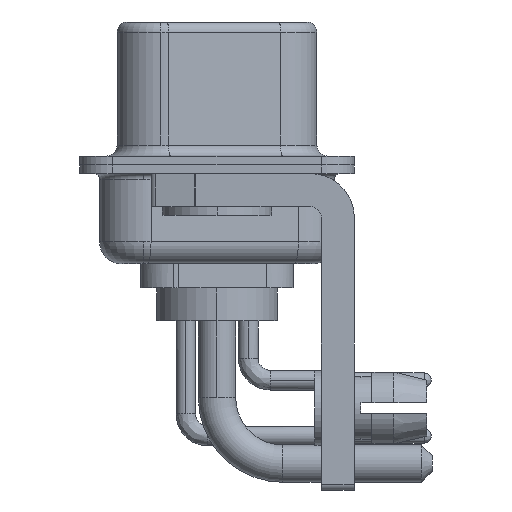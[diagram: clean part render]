
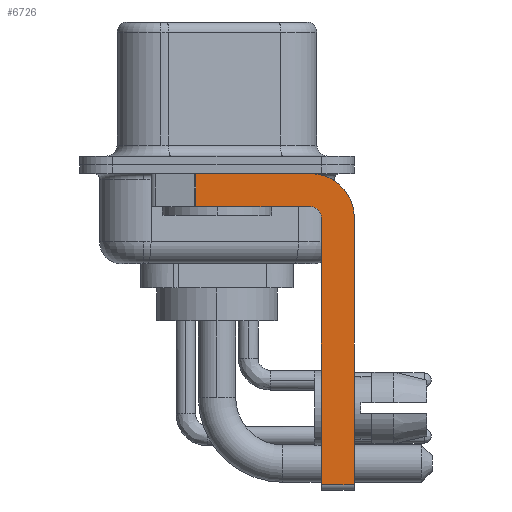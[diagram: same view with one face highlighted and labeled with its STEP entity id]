
A CAD part, left-side view. The second image highlights one B-rep face of the part: STEP entity #6726.
In plain terms, the highlighted planar face has unit normal (-1, 0, 0).
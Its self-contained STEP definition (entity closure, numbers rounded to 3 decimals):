
#48 = DIRECTION ( 'NONE',  ( 0., -1., 0. ) ) ;
#87 = PLANE ( 'NONE',  #20962 ) ;
#122 = CARTESIAN_POINT ( 'NONE',  ( -2.9, -4.75, -2.4 ) ) ;
#346 = EDGE_CURVE ( 'NONE', #7438, #11156, #21705, .T. ) ;
#1216 = VERTEX_POINT ( 'NONE', #8095 ) ;
#1257 = CARTESIAN_POINT ( 'NONE',  ( -2.9, 0.978, -0.4 ) ) ;
#1476 = CARTESIAN_POINT ( 'NONE',  ( -2.9, -4.25, -2.4 ) ) ;
#1840 = DIRECTION ( 'NONE',  ( 1., 0., 0. ) ) ;
#2234 = FACE_OUTER_BOUND ( 'NONE', #18612, .T. ) ;
#3149 = VERTEX_POINT ( 'NONE', #19498 ) ;
#3639 = CARTESIAN_POINT ( 'NONE',  ( -2.9, 0.978, -1.9 ) ) ;
#5257 = ORIENTED_EDGE ( 'NONE', *, *, #14508, .F. ) ;
#5869 = EDGE_CURVE ( 'NONE', #7438, #3149, #22222, .T. ) ;
#6054 = EDGE_CURVE ( 'NONE', #3149, #11250, #22698, .T. ) ;
#6210 = VERTEX_POINT ( 'NONE', #122 ) ;
#6679 = ORIENTED_EDGE ( 'NONE', *, *, #24020, .F. ) ;
#6726 = ADVANCED_FACE ( 'NONE', ( #2234 ), #87, .F. ) ;
#7407 = VECTOR ( 'NONE', #7600, 1000. ) ;
#7438 = VERTEX_POINT ( 'NONE', #1257 ) ;
#7576 = LINE ( 'NONE', #26226, #7935 ) ;
#7600 = DIRECTION ( 'NONE',  ( 0., 1., 0. ) ) ;
#7700 = CIRCLE ( 'NONE', #17254, 0.5 ) ;
#7927 = CARTESIAN_POINT ( 'NONE',  ( -2.9, 3., -0.4 ) ) ;
#7935 = VECTOR ( 'NONE', #20372, 1000. ) ;
#8095 = CARTESIAN_POINT ( 'NONE',  ( -2.9, -6.25, -14.55 ) ) ;
#8787 = CARTESIAN_POINT ( 'NONE',  ( -2.9, -6.25, -2.4 ) ) ;
#9213 = AXIS2_PLACEMENT_3D ( 'NONE', #1476, #23934, #15890 ) ;
#10124 = CARTESIAN_POINT ( 'NONE',  ( -2.9, -4.75, -14.55 ) ) ;
#10444 = CARTESIAN_POINT ( 'NONE',  ( -2.9, -6.25, -2.4 ) ) ;
#11156 = VERTEX_POINT ( 'NONE', #3639 ) ;
#11174 = CARTESIAN_POINT ( 'NONE',  ( -2.9, -4.25, -1.9 ) ) ;
#11250 = VERTEX_POINT ( 'NONE', #10444 ) ;
#11798 = ORIENTED_EDGE ( 'NONE', *, *, #16405, .F. ) ;
#12234 = VECTOR ( 'NONE', #48, 1000. ) ;
#13249 = CARTESIAN_POINT ( 'NONE',  ( -2.9, 0.978, -1.9 ) ) ;
#14508 = EDGE_CURVE ( 'NONE', #6210, #23359, #7700, .T. ) ;
#14541 = LINE ( 'NONE', #18670, #16910 ) ;
#14832 = ORIENTED_EDGE ( 'NONE', *, *, #6054, .F. ) ;
#15890 = DIRECTION ( 'NONE',  ( 0., 0., -1. ) ) ;
#16405 = EDGE_CURVE ( 'NONE', #24233, #6210, #14541, .T. ) ;
#16554 = ORIENTED_EDGE ( 'NONE', *, *, #346, .T. ) ;
#16667 = DIRECTION ( 'NONE',  ( 0., 0., -1. ) ) ;
#16910 = VECTOR ( 'NONE', #23007, 1000. ) ;
#17254 = AXIS2_PLACEMENT_3D ( 'NONE', #18342, #18069, #22569 ) ;
#17603 = ORIENTED_EDGE ( 'NONE', *, *, #25861, .T. ) ;
#18069 = DIRECTION ( 'NONE',  ( -1., 0., 0. ) ) ;
#18144 = VECTOR ( 'NONE', #19416, 1000. ) ;
#18342 = CARTESIAN_POINT ( 'NONE',  ( -2.9, -4.25, -2.4 ) ) ;
#18612 = EDGE_LOOP ( 'NONE', ( #25729, #16554, #6679, #5257, #11798, #17603, #20588, #14832 ) ) ;
#18670 = CARTESIAN_POINT ( 'NONE',  ( -2.9, -4.75, -14.8 ) ) ;
#19051 = EDGE_CURVE ( 'NONE', #11250, #1216, #21045, .T. ) ;
#19416 = DIRECTION ( 'NONE',  ( 0., 0., -1. ) ) ;
#19498 = CARTESIAN_POINT ( 'NONE',  ( -2.9, -4.25, -0.4 ) ) ;
#20372 = DIRECTION ( 'NONE',  ( 0., -1., 0. ) ) ;
#20490 = CARTESIAN_POINT ( 'NONE',  ( -2.9, -4.25, -2.4 ) ) ;
#20588 = ORIENTED_EDGE ( 'NONE', *, *, #19051, .F. ) ;
#20962 = AXIS2_PLACEMENT_3D ( 'NONE', #20490, #1840, #16667 ) ;
#21045 = LINE ( 'NONE', #8787, #18144 ) ;
#21520 = VECTOR ( 'NONE', #25524, 1000. ) ;
#21705 = LINE ( 'NONE', #13249, #21520 ) ;
#22222 = LINE ( 'NONE', #7927, #12234 ) ;
#22569 = DIRECTION ( 'NONE',  ( 0., 0., 1. ) ) ;
#22698 = CIRCLE ( 'NONE', #9213, 2. ) ;
#23007 = DIRECTION ( 'NONE',  ( 0., 0., 1. ) ) ;
#23359 = VERTEX_POINT ( 'NONE', #11174 ) ;
#23934 = DIRECTION ( 'NONE',  ( 1., 0., 0. ) ) ;
#24020 = EDGE_CURVE ( 'NONE', #23359, #11156, #24073, .T. ) ;
#24073 = LINE ( 'NONE', #26252, #7407 ) ;
#24233 = VERTEX_POINT ( 'NONE', #10124 ) ;
#25524 = DIRECTION ( 'NONE',  ( 0., 0., -1. ) ) ;
#25729 = ORIENTED_EDGE ( 'NONE', *, *, #5869, .F. ) ;
#25861 = EDGE_CURVE ( 'NONE', #24233, #1216, #7576, .T. ) ;
#26226 = CARTESIAN_POINT ( 'NONE',  ( -2.9, -4.25, -14.55 ) ) ;
#26252 = CARTESIAN_POINT ( 'NONE',  ( -2.9, -4.25, -1.9 ) ) ;
